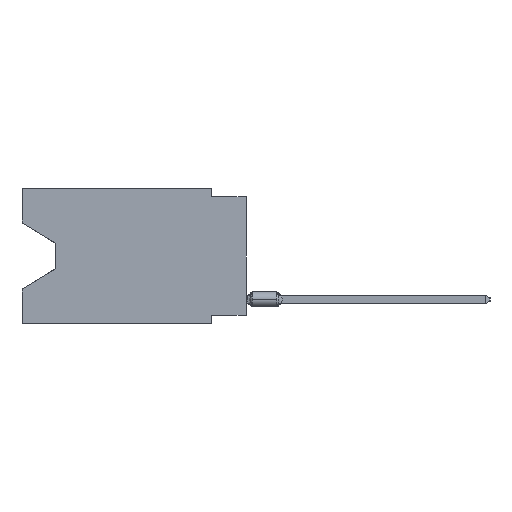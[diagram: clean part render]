
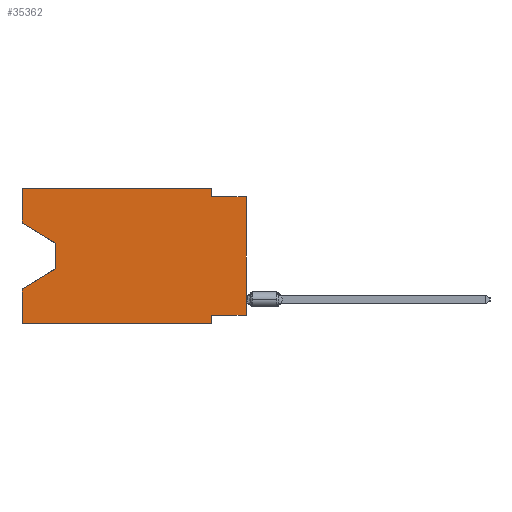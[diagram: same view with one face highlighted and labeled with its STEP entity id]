
A CAD part, left-side view. The second image highlights one B-rep face of the part: STEP entity #35362.
In plain terms, the highlighted planar face has unit normal (-1, 0, 0).
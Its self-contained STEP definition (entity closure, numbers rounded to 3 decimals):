
#258 = CARTESIAN_POINT ( 'NONE',  ( 0., 2.54, 0. ) ) ;
#1427 = CARTESIAN_POINT ( 'NONE',  ( 0., 16.383, 0. ) ) ;
#2366 = ORIENTED_EDGE ( 'NONE', *, *, #10672, .F. ) ;
#2534 = ORIENTED_EDGE ( 'NONE', *, *, #5590, .T. ) ;
#2714 = ORIENTED_EDGE ( 'NONE', *, *, #33137, .F. ) ;
#4896 = CARTESIAN_POINT ( 'NONE',  ( 0., 16.383, -7.36 ) ) ;
#5013 = DIRECTION ( 'NONE',  ( 0., -1., 0. ) ) ;
#5513 = DIRECTION ( 'NONE',  ( 0., 0., -1. ) ) ;
#5561 = VERTEX_POINT ( 'NONE', #22358 ) ;
#5590 = EDGE_CURVE ( 'NONE', #48627, #49921, #18638, .T. ) ;
#6487 = EDGE_CURVE ( 'NONE', #8258, #16383, #36408, .T. ) ;
#7343 = VECTOR ( 'NONE', #33564, 1000. ) ;
#7412 = CARTESIAN_POINT ( 'NONE',  ( 0., 2.54, -9.271 ) ) ;
#7492 = VECTOR ( 'NONE', #13345, 1000. ) ;
#7656 = VECTOR ( 'NONE', #41163, 1000. ) ;
#7808 = FACE_OUTER_BOUND ( 'NONE', #28330, .T. ) ;
#8258 = VERTEX_POINT ( 'NONE', #19263 ) ;
#8392 = VECTOR ( 'NONE', #38580, 1000. ) ;
#8460 = LINE ( 'NONE', #13217, #32634 ) ;
#8618 = ORIENTED_EDGE ( 'NONE', *, *, #49177, .F. ) ;
#9892 = EDGE_CURVE ( 'NONE', #49888, #8258, #8460, .T. ) ;
#10672 = EDGE_CURVE ( 'NONE', #15395, #24436, #43714, .T. ) ;
#11199 = ORIENTED_EDGE ( 'NONE', *, *, #17836, .F. ) ;
#13217 = CARTESIAN_POINT ( 'NONE',  ( 0., 16.383, 0. ) ) ;
#13345 = DIRECTION ( 'NONE',  ( 0., -1., 0. ) ) ;
#13462 = VECTOR ( 'NONE', #17563, 1000. ) ;
#14493 = CARTESIAN_POINT ( 'NONE',  ( 0., 16.383, -2.546 ) ) ;
#15395 = VERTEX_POINT ( 'NONE', #7412 ) ;
#15449 = CARTESIAN_POINT ( 'NONE',  ( 0., 13.97, -4.013 ) ) ;
#15788 = EDGE_CURVE ( 'NONE', #20750, #15395, #42071, .T. ) ;
#16379 = LINE ( 'NONE', #16634, #21729 ) ;
#16383 = VERTEX_POINT ( 'NONE', #44360 ) ;
#16634 = CARTESIAN_POINT ( 'NONE',  ( 0., 0., -0.635 ) ) ;
#16970 = EDGE_CURVE ( 'NONE', #5561, #24436, #21626, .T. ) ;
#17563 = DIRECTION ( 'NONE',  ( 0., 0., 1. ) ) ;
#17836 = EDGE_CURVE ( 'NONE', #5561, #49921, #32984, .T. ) ;
#17883 = CARTESIAN_POINT ( 'NONE',  ( 0., 16.383, -9.906 ) ) ;
#18477 = ORIENTED_EDGE ( 'NONE', *, *, #26663, .T. ) ;
#18487 = EDGE_CURVE ( 'NONE', #20750, #35284, #28085, .T. ) ;
#18638 = LINE ( 'NONE', #38835, #8392 ) ;
#19263 = CARTESIAN_POINT ( 'NONE',  ( 0., 2.54, 0. ) ) ;
#19588 = DIRECTION ( 'NONE',  ( 0., 0., 1. ) ) ;
#20750 = VERTEX_POINT ( 'NONE', #39652 ) ;
#21550 = DIRECTION ( 'NONE',  ( 0., 0., 1. ) ) ;
#21626 = LINE ( 'NONE', #17883, #7492 ) ;
#21729 = VECTOR ( 'NONE', #49043, 1000. ) ;
#22057 = ORIENTED_EDGE ( 'NONE', *, *, #38466, .T. ) ;
#22358 = CARTESIAN_POINT ( 'NONE',  ( 0., 16.383, -9.906 ) ) ;
#22686 = VERTEX_POINT ( 'NONE', #15449 ) ;
#24436 = VERTEX_POINT ( 'NONE', #49619 ) ;
#24500 = DIRECTION ( 'NONE',  ( 0., 0., -1. ) ) ;
#24528 = AXIS2_PLACEMENT_3D ( 'NONE', #52175, #32267, #44473 ) ;
#25292 = LINE ( 'NONE', #45742, #13462 ) ;
#25729 = CARTESIAN_POINT ( 'NONE',  ( 0., 13.97, -4.013 ) ) ;
#26415 = ORIENTED_EDGE ( 'NONE', *, *, #16970, .T. ) ;
#26663 = EDGE_CURVE ( 'NONE', #32626, #22686, #32518, .T. ) ;
#27219 = VECTOR ( 'NONE', #19588, 1000. ) ;
#28085 = LINE ( 'NONE', #48267, #27219 ) ;
#28330 = EDGE_LOOP ( 'NONE', ( #18477, #22057, #2534, #11199, #26415, #2366, #49598, #32912, #2714, #30743, #51686, #8618 ) ) ;
#30743 = ORIENTED_EDGE ( 'NONE', *, *, #6487, .F. ) ;
#31237 = CARTESIAN_POINT ( 'NONE',  ( 0., 2.54, -9.906 ) ) ;
#32267 = DIRECTION ( 'NONE',  ( 1., 0., 0. ) ) ;
#32518 = LINE ( 'NONE', #40226, #41243 ) ;
#32626 = VERTEX_POINT ( 'NONE', #14493 ) ;
#32634 = VECTOR ( 'NONE', #5013, 1000. ) ;
#32912 = ORIENTED_EDGE ( 'NONE', *, *, #18487, .T. ) ;
#32984 = LINE ( 'NONE', #41751, #37354 ) ;
#33137 = EDGE_CURVE ( 'NONE', #16383, #35284, #16379, .T. ) ;
#33564 = DIRECTION ( 'NONE',  ( 0., 1., 0. ) ) ;
#35284 = VERTEX_POINT ( 'NONE', #44730 ) ;
#35362 = ADVANCED_FACE ( 'NONE', ( #7808 ), #36775, .F. ) ;
#36408 = LINE ( 'NONE', #258, #7656 ) ;
#36775 = PLANE ( 'NONE',  #24528 ) ;
#36789 = CARTESIAN_POINT ( 'NONE',  ( 0., 13.97, -5.893 ) ) ;
#37354 = VECTOR ( 'NONE', #21550, 1000. ) ;
#38199 = LINE ( 'NONE', #25729, #50701 ) ;
#38466 = EDGE_CURVE ( 'NONE', #22686, #48627, #38199, .T. ) ;
#38580 = DIRECTION ( 'NONE',  ( 0., 0.855, -0.519 ) ) ;
#38835 = CARTESIAN_POINT ( 'NONE',  ( 0., 13.97, -5.893 ) ) ;
#39652 = CARTESIAN_POINT ( 'NONE',  ( 0., 0., -9.271 ) ) ;
#40226 = CARTESIAN_POINT ( 'NONE',  ( 0., 16.383, -2.546 ) ) ;
#41034 = VECTOR ( 'NONE', #24500, 1000. ) ;
#41163 = DIRECTION ( 'NONE',  ( 0., 0., -1. ) ) ;
#41243 = VECTOR ( 'NONE', #52422, 1000. ) ;
#41751 = CARTESIAN_POINT ( 'NONE',  ( 0., 16.383, 0. ) ) ;
#42071 = LINE ( 'NONE', #49763, #7343 ) ;
#43714 = LINE ( 'NONE', #31237, #41034 ) ;
#44360 = CARTESIAN_POINT ( 'NONE',  ( 0., 2.54, -0.635 ) ) ;
#44473 = DIRECTION ( 'NONE',  ( 0., 0., -1. ) ) ;
#44730 = CARTESIAN_POINT ( 'NONE',  ( 0., 0., -0.635 ) ) ;
#45742 = CARTESIAN_POINT ( 'NONE',  ( 0., 16.383, 0. ) ) ;
#48267 = CARTESIAN_POINT ( 'NONE',  ( 0., 0., 0. ) ) ;
#48627 = VERTEX_POINT ( 'NONE', #36789 ) ;
#49043 = DIRECTION ( 'NONE',  ( 0., -1., 0. ) ) ;
#49177 = EDGE_CURVE ( 'NONE', #32626, #49888, #25292, .T. ) ;
#49598 = ORIENTED_EDGE ( 'NONE', *, *, #15788, .F. ) ;
#49619 = CARTESIAN_POINT ( 'NONE',  ( 0., 2.54, -9.906 ) ) ;
#49763 = CARTESIAN_POINT ( 'NONE',  ( 0., 0., -9.271 ) ) ;
#49888 = VERTEX_POINT ( 'NONE', #1427 ) ;
#49921 = VERTEX_POINT ( 'NONE', #4896 ) ;
#50701 = VECTOR ( 'NONE', #5513, 1000. ) ;
#51686 = ORIENTED_EDGE ( 'NONE', *, *, #9892, .F. ) ;
#52175 = CARTESIAN_POINT ( 'NONE',  ( 0., 16.383, 0. ) ) ;
#52422 = DIRECTION ( 'NONE',  ( 0., -0.855, -0.519 ) ) ;
